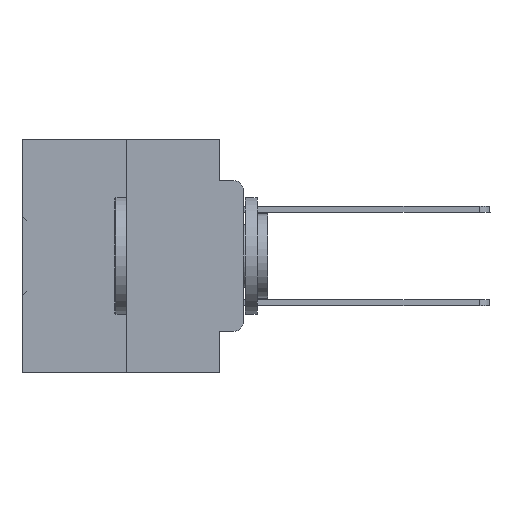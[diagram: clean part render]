
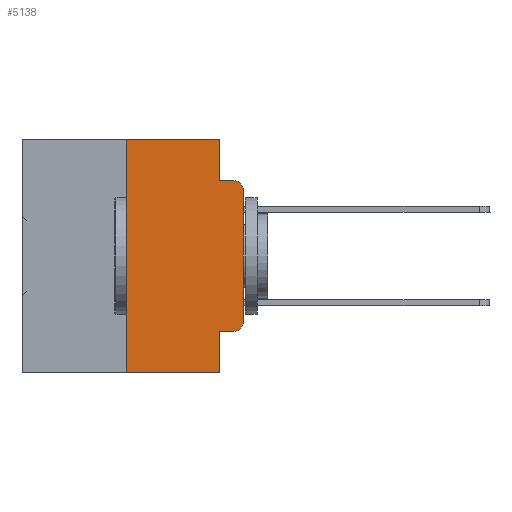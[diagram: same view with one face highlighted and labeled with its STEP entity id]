
A CAD part, left-side view. The second image highlights one B-rep face of the part: STEP entity #5138.
In plain terms, the highlighted planar face has unit normal (-1, 0, 0).
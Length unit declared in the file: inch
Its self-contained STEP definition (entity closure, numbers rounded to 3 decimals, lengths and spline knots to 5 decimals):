
#415 = VERTEX_POINT ( 'NONE', #6512 ) ;
#584 = CARTESIAN_POINT ( 'NONE',  ( 0., 0.02, -0.0885 ) ) ;
#819 = CIRCLE ( 'NONE', #18423, 0.02 ) ;
#852 = CARTESIAN_POINT ( 'NONE',  ( 0., 0., 0. ) ) ;
#1063 = DIRECTION ( 'NONE',  ( 0., -1., 0. ) ) ;
#1245 = DIRECTION ( 'NONE',  ( 0., 0., -1. ) ) ;
#1471 = EDGE_CURVE ( 'NONE', #415, #22983, #3068, .T. ) ;
#2902 = VERTEX_POINT ( 'NONE', #26537 ) ;
#3068 = LINE ( 'NONE', #852, #17211 ) ;
#3371 = AXIS2_PLACEMENT_3D ( 'NONE', #30913, #4818, #31033 ) ;
#3805 = LINE ( 'NONE', #32713, #6076 ) ;
#4001 = VERTEX_POINT ( 'NONE', #584 ) ;
#4355 = EDGE_LOOP ( 'NONE', ( #11803, #16839, #10119, #4817, #10590, #34935, #18846, #36532, #14316, #15706 ) ) ;
#4530 = LINE ( 'NONE', #31801, #24649 ) ;
#4817 = ORIENTED_EDGE ( 'NONE', *, *, #13757, .F. ) ;
#4818 = DIRECTION ( 'NONE',  ( 1., 0., 0. ) ) ;
#5123 = CARTESIAN_POINT ( 'NONE',  ( 0., 0.25, 0. ) ) ;
#5138 = ADVANCED_FACE ( 'NONE', ( #14731 ), #28251, .F. ) ;
#5443 = CARTESIAN_POINT ( 'NONE',  ( 0., 0.051, 0. ) ) ;
#6076 = VECTOR ( 'NONE', #1063, 39.37008 ) ;
#6512 = CARTESIAN_POINT ( 'NONE',  ( 0., 0., -0.3915 ) ) ;
#6707 = VERTEX_POINT ( 'NONE', #5443 ) ;
#6935 = CARTESIAN_POINT ( 'NONE',  ( 0., 0.051, -0.4115 ) ) ;
#9587 = DIRECTION ( 'NONE',  ( 0., 0., -1. ) ) ;
#10119 = ORIENTED_EDGE ( 'NONE', *, *, #20738, .F. ) ;
#10345 = CARTESIAN_POINT ( 'NONE',  ( 0., 0., -0.1085 ) ) ;
#10525 = EDGE_CURVE ( 'NONE', #14246, #415, #819, .T. ) ;
#10590 = ORIENTED_EDGE ( 'NONE', *, *, #32221, .F. ) ;
#11110 = CARTESIAN_POINT ( 'NONE',  ( 0., 0.051, -0.5 ) ) ;
#11803 = ORIENTED_EDGE ( 'NONE', *, *, #1471, .T. ) ;
#12904 = EDGE_CURVE ( 'NONE', #18602, #14246, #3805, .T. ) ;
#13137 = CIRCLE ( 'NONE', #32271, 0.02 ) ;
#13620 = CARTESIAN_POINT ( 'NONE',  ( 0., 0.473, -0.5 ) ) ;
#13757 = EDGE_CURVE ( 'NONE', #6707, #31607, #16845, .T. ) ;
#14246 = VERTEX_POINT ( 'NONE', #36737 ) ;
#14316 = ORIENTED_EDGE ( 'NONE', *, *, #12904, .T. ) ;
#14731 = FACE_OUTER_BOUND ( 'NONE', #4355, .T. ) ;
#14819 = LINE ( 'NONE', #13620, #24874 ) ;
#15706 = ORIENTED_EDGE ( 'NONE', *, *, #10525, .T. ) ;
#16801 = LINE ( 'NONE', #24996, #29071 ) ;
#16839 = ORIENTED_EDGE ( 'NONE', *, *, #34561, .T. ) ;
#16845 = LINE ( 'NONE', #23141, #27800 ) ;
#17211 = VECTOR ( 'NONE', #24477, 39.37008 ) ;
#17700 = LINE ( 'NONE', #30010, #19987 ) ;
#18423 = AXIS2_PLACEMENT_3D ( 'NONE', #26790, #27307, #9587 ) ;
#18602 = VERTEX_POINT ( 'NONE', #6935 ) ;
#18846 = ORIENTED_EDGE ( 'NONE', *, *, #23574, .T. ) ;
#19987 = VECTOR ( 'NONE', #1245, 39.37008 ) ;
#20738 = EDGE_CURVE ( 'NONE', #31607, #4001, #4530, .T. ) ;
#21745 = EDGE_CURVE ( 'NONE', #18602, #31454, #17700, .T. ) ;
#22059 = DIRECTION ( 'NONE',  ( 0., -1., 0. ) ) ;
#22983 = VERTEX_POINT ( 'NONE', #10345 ) ;
#23079 = CARTESIAN_POINT ( 'NONE',  ( 0., 0.25, 0. ) ) ;
#23141 = CARTESIAN_POINT ( 'NONE',  ( 0., 0.051, 0. ) ) ;
#23249 = DIRECTION ( 'NONE',  ( 0., -1., 0. ) ) ;
#23566 = DIRECTION ( 'NONE',  ( -1., 0., 0. ) ) ;
#23574 = EDGE_CURVE ( 'NONE', #2902, #31454, #14819, .T. ) ;
#24477 = DIRECTION ( 'NONE',  ( 0., 0., 1. ) ) ;
#24649 = VECTOR ( 'NONE', #23249, 39.37008 ) ;
#24874 = VECTOR ( 'NONE', #33940, 39.37008 ) ;
#24996 = CARTESIAN_POINT ( 'NONE',  ( 0., 0.473, 0. ) ) ;
#25194 = DIRECTION ( 'NONE',  ( 0., 0., 1. ) ) ;
#26537 = CARTESIAN_POINT ( 'NONE',  ( 0., 0.25, -0.5 ) ) ;
#26698 = CARTESIAN_POINT ( 'NONE',  ( 0., 0.02, -0.1085 ) ) ;
#26790 = CARTESIAN_POINT ( 'NONE',  ( 0., 0.02, -0.3915 ) ) ;
#27307 = DIRECTION ( 'NONE',  ( -1., 0., 0. ) ) ;
#27737 = EDGE_CURVE ( 'NONE', #2902, #36836, #29844, .T. ) ;
#27800 = VECTOR ( 'NONE', #31820, 39.37008 ) ;
#28251 = PLANE ( 'NONE',  #3371 ) ;
#29071 = VECTOR ( 'NONE', #22059, 39.37008 ) ;
#29844 = LINE ( 'NONE', #5123, #33003 ) ;
#30010 = CARTESIAN_POINT ( 'NONE',  ( 0., 0.051, 0. ) ) ;
#30913 = CARTESIAN_POINT ( 'NONE',  ( 0., 0.473, 0. ) ) ;
#31033 = DIRECTION ( 'NONE',  ( 0., 0., -1. ) ) ;
#31454 = VERTEX_POINT ( 'NONE', #11110 ) ;
#31607 = VERTEX_POINT ( 'NONE', #32636 ) ;
#31801 = CARTESIAN_POINT ( 'NONE',  ( 0., 0.051, -0.0885 ) ) ;
#31820 = DIRECTION ( 'NONE',  ( 0., 0., -1. ) ) ;
#32221 = EDGE_CURVE ( 'NONE', #36836, #6707, #16801, .T. ) ;
#32271 = AXIS2_PLACEMENT_3D ( 'NONE', #26698, #23566, #32489 ) ;
#32489 = DIRECTION ( 'NONE',  ( 0., 0., -1. ) ) ;
#32636 = CARTESIAN_POINT ( 'NONE',  ( 0., 0.051, -0.0885 ) ) ;
#32713 = CARTESIAN_POINT ( 'NONE',  ( 0., 0.051, -0.4115 ) ) ;
#33003 = VECTOR ( 'NONE', #25194, 39.37008 ) ;
#33940 = DIRECTION ( 'NONE',  ( 0., -1., 0. ) ) ;
#34561 = EDGE_CURVE ( 'NONE', #22983, #4001, #13137, .T. ) ;
#34935 = ORIENTED_EDGE ( 'NONE', *, *, #27737, .F. ) ;
#36532 = ORIENTED_EDGE ( 'NONE', *, *, #21745, .F. ) ;
#36737 = CARTESIAN_POINT ( 'NONE',  ( 0., 0.02, -0.4115 ) ) ;
#36836 = VERTEX_POINT ( 'NONE', #23079 ) ;
